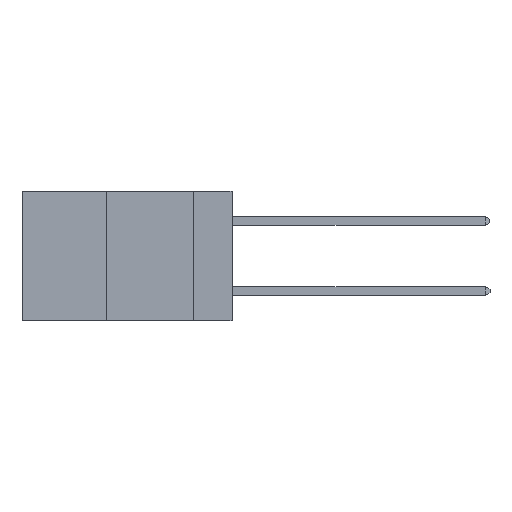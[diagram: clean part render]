
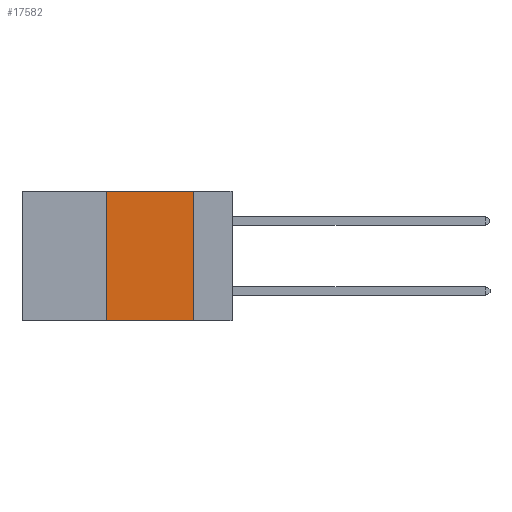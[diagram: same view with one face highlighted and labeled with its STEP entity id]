
A CAD part, left-side view. The second image highlights one B-rep face of the part: STEP entity #17582.
In plain terms, the highlighted planar face has unit normal (-1, 0, 0).
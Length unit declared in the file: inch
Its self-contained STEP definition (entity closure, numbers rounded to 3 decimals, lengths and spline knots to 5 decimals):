
#124 = CARTESIAN_POINT ( 'NONE',  ( 0., 0.6, 0. ) ) ;
#241 = ORIENTED_EDGE ( 'NONE', *, *, #9833, .T. ) ;
#584 = LINE ( 'NONE', #5471, #4860 ) ;
#1083 = EDGE_CURVE ( 'NONE', #17901, #15748, #584, .T. ) ;
#1631 = DIRECTION ( 'NONE',  ( 0., 0., -1. ) ) ;
#1972 = CARTESIAN_POINT ( 'NONE',  ( 0., 0.11, 0. ) ) ;
#2197 = FACE_OUTER_BOUND ( 'NONE', #15044, .T. ) ;
#2744 = LINE ( 'NONE', #7953, #9584 ) ;
#3044 = VERTEX_POINT ( 'NONE', #16651 ) ;
#4860 = VECTOR ( 'NONE', #10560, 39.37008 ) ;
#4880 = CARTESIAN_POINT ( 'NONE',  ( 0., 0.6, -0.37 ) ) ;
#4910 = LINE ( 'NONE', #4880, #11412 ) ;
#5195 = CARTESIAN_POINT ( 'NONE',  ( 0., 0.36, 0. ) ) ;
#5471 = CARTESIAN_POINT ( 'NONE',  ( 0., 0.36, 0. ) ) ;
#6424 = VERTEX_POINT ( 'NONE', #1972 ) ;
#6662 = ORIENTED_EDGE ( 'NONE', *, *, #15366, .F. ) ;
#7766 = CARTESIAN_POINT ( 'NONE',  ( 0., 0.36, -0.37 ) ) ;
#7953 = CARTESIAN_POINT ( 'NONE',  ( 0., 0.6, 0. ) ) ;
#8518 = PLANE ( 'NONE',  #13322 ) ;
#9584 = VECTOR ( 'NONE', #14913, 39.37008 ) ;
#9833 = EDGE_CURVE ( 'NONE', #17901, #3044, #4910, .T. ) ;
#9933 = DIRECTION ( 'NONE',  ( 1., 0., 0. ) ) ;
#10267 = VECTOR ( 'NONE', #14236, 39.37008 ) ;
#10560 = DIRECTION ( 'NONE',  ( 0., 0., 1. ) ) ;
#10710 = LINE ( 'NONE', #12895, #10267 ) ;
#10716 = ORIENTED_EDGE ( 'NONE', *, *, #14923, .F. ) ;
#11412 = VECTOR ( 'NONE', #13156, 39.37008 ) ;
#12895 = CARTESIAN_POINT ( 'NONE',  ( 0., 0.11, 0. ) ) ;
#13156 = DIRECTION ( 'NONE',  ( 0., -1., 0. ) ) ;
#13322 = AXIS2_PLACEMENT_3D ( 'NONE', #124, #9933, #1631 ) ;
#14236 = DIRECTION ( 'NONE',  ( 0., 0., -1. ) ) ;
#14913 = DIRECTION ( 'NONE',  ( 0., -1., 0. ) ) ;
#14923 = EDGE_CURVE ( 'NONE', #15748, #6424, #2744, .T. ) ;
#15044 = EDGE_LOOP ( 'NONE', ( #6662, #10716, #16536, #241 ) ) ;
#15366 = EDGE_CURVE ( 'NONE', #6424, #3044, #10710, .T. ) ;
#15748 = VERTEX_POINT ( 'NONE', #5195 ) ;
#16536 = ORIENTED_EDGE ( 'NONE', *, *, #1083, .F. ) ;
#16651 = CARTESIAN_POINT ( 'NONE',  ( 0., 0.11, -0.37 ) ) ;
#17582 = ADVANCED_FACE ( 'NONE', ( #2197 ), #8518, .F. ) ;
#17901 = VERTEX_POINT ( 'NONE', #7766 ) ;
